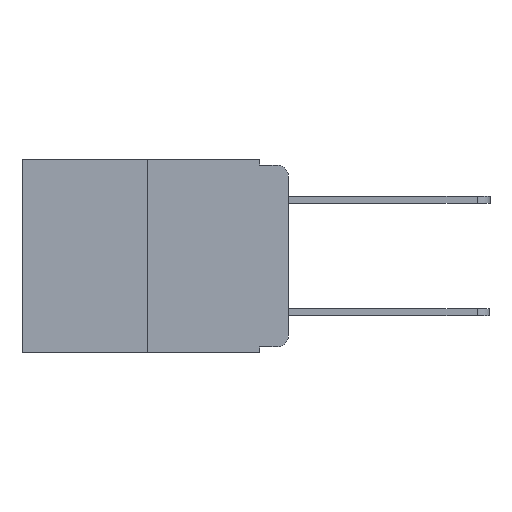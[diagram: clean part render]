
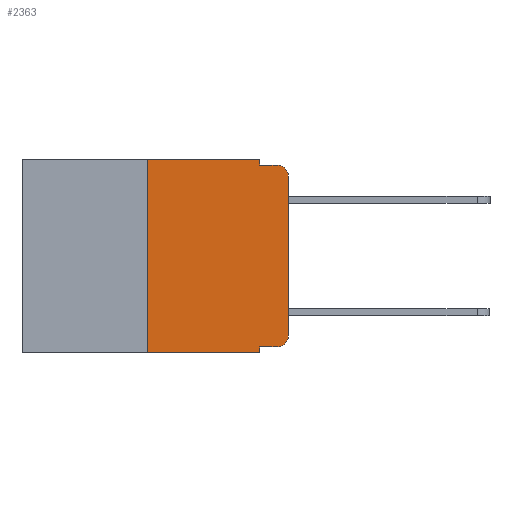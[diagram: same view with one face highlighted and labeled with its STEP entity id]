
A CAD part, left-side view. The second image highlights one B-rep face of the part: STEP entity #2363.
In plain terms, the highlighted planar face has unit normal (-1, 0, 0).
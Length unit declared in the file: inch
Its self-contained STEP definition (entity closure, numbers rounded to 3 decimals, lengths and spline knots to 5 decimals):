
#89 = CARTESIAN_POINT ( 'NONE',  ( 0., 0.051, -0.333 ) ) ;
#152 = ORIENTED_EDGE ( 'NONE', *, *, #4042, .F. ) ;
#178 = DIRECTION ( 'NONE',  ( -1., 0., 0. ) ) ;
#197 = LINE ( 'NONE', #7037, #9937 ) ;
#241 = VECTOR ( 'NONE', #9816, 39.37008 ) ;
#544 = EDGE_CURVE ( 'NONE', #943, #4559, #9463, .T. ) ;
#662 = LINE ( 'NONE', #4929, #1022 ) ;
#840 = CIRCLE ( 'NONE', #10799, 0.02 ) ;
#892 = CARTESIAN_POINT ( 'NONE',  ( 0., 0.473, -0.343 ) ) ;
#908 = CARTESIAN_POINT ( 'NONE',  ( 0., 0.02, -0.333 ) ) ;
#943 = VERTEX_POINT ( 'NONE', #12039 ) ;
#1022 = VECTOR ( 'NONE', #5975, 39.37008 ) ;
#1100 = VERTEX_POINT ( 'NONE', #9265 ) ;
#1186 = VERTEX_POINT ( 'NONE', #7700 ) ;
#1202 = VERTEX_POINT ( 'NONE', #908 ) ;
#1264 = EDGE_CURVE ( 'NONE', #10830, #1186, #840, .T. ) ;
#1956 = DIRECTION ( 'NONE',  ( 0., 0., -1. ) ) ;
#2053 = CARTESIAN_POINT ( 'NONE',  ( 0., 0., -0.313 ) ) ;
#2106 = VECTOR ( 'NONE', #7248, 39.37008 ) ;
#2107 = DIRECTION ( 'NONE',  ( 0., 0., 1. ) ) ;
#2241 = CARTESIAN_POINT ( 'NONE',  ( 0., 0.02, -0.03 ) ) ;
#2311 = VECTOR ( 'NONE', #10447, 39.37008 ) ;
#2363 = ADVANCED_FACE ( 'NONE', ( #5228 ), #12243, .F. ) ;
#2385 = EDGE_CURVE ( 'NONE', #7350, #4559, #12242, .T. ) ;
#2438 = DIRECTION ( 'NONE',  ( 0., 0., 1. ) ) ;
#2677 = ORIENTED_EDGE ( 'NONE', *, *, #10457, .T. ) ;
#2814 = CARTESIAN_POINT ( 'NONE',  ( 0., 0.051, 0. ) ) ;
#2967 = ORIENTED_EDGE ( 'NONE', *, *, #4863, .F. ) ;
#3004 = CARTESIAN_POINT ( 'NONE',  ( 0., 0., -0.03 ) ) ;
#3276 = ORIENTED_EDGE ( 'NONE', *, *, #10829, .T. ) ;
#3390 = DIRECTION ( 'NONE',  ( 0., -1., 0. ) ) ;
#3733 = VERTEX_POINT ( 'NONE', #10480 ) ;
#3808 = VERTEX_POINT ( 'NONE', #2053 ) ;
#3965 = EDGE_CURVE ( 'NONE', #943, #1202, #10266, .T. ) ;
#4001 = ORIENTED_EDGE ( 'NONE', *, *, #544, .F. ) ;
#4042 = EDGE_CURVE ( 'NONE', #3733, #5033, #4704, .T. ) ;
#4559 = VERTEX_POINT ( 'NONE', #4950 ) ;
#4704 = LINE ( 'NONE', #8145, #2106 ) ;
#4743 = DIRECTION ( 'NONE',  ( -1., 0., 0. ) ) ;
#4863 = EDGE_CURVE ( 'NONE', #1100, #3733, #7452, .T. ) ;
#4888 = CARTESIAN_POINT ( 'NONE',  ( 0., 0.473, 0. ) ) ;
#4929 = CARTESIAN_POINT ( 'NONE',  ( 0., 0.051, -0.01 ) ) ;
#4950 = CARTESIAN_POINT ( 'NONE',  ( 0., 0.051, -0.343 ) ) ;
#5033 = VERTEX_POINT ( 'NONE', #5671 ) ;
#5228 = FACE_OUTER_BOUND ( 'NONE', #5438, .T. ) ;
#5269 = ORIENTED_EDGE ( 'NONE', *, *, #12322, .F. ) ;
#5438 = EDGE_LOOP ( 'NONE', ( #2677, #7539, #5269, #152, #2967, #8085, #8780, #4001, #7242, #3276 ) ) ;
#5595 = DIRECTION ( 'NONE',  ( 0., 0., -1. ) ) ;
#5671 = CARTESIAN_POINT ( 'NONE',  ( 0., 0.051, -0.01 ) ) ;
#5767 = LINE ( 'NONE', #8212, #6094 ) ;
#5975 = DIRECTION ( 'NONE',  ( 0., -1., 0. ) ) ;
#6094 = VECTOR ( 'NONE', #2438, 39.37008 ) ;
#6376 = CARTESIAN_POINT ( 'NONE',  ( 0., 0.473, 0. ) ) ;
#6902 = DIRECTION ( 'NONE',  ( 0., 0., -1. ) ) ;
#7037 = CARTESIAN_POINT ( 'NONE',  ( 0., 0., 0. ) ) ;
#7242 = ORIENTED_EDGE ( 'NONE', *, *, #3965, .T. ) ;
#7248 = DIRECTION ( 'NONE',  ( 0., 0., -1. ) ) ;
#7350 = VERTEX_POINT ( 'NONE', #8929 ) ;
#7452 = LINE ( 'NONE', #6376, #11904 ) ;
#7539 = ORIENTED_EDGE ( 'NONE', *, *, #1264, .T. ) ;
#7700 = CARTESIAN_POINT ( 'NONE',  ( 0., 0.02, -0.01 ) ) ;
#7986 = CIRCLE ( 'NONE', #11309, 0.02 ) ;
#8085 = ORIENTED_EDGE ( 'NONE', *, *, #11654, .F. ) ;
#8145 = CARTESIAN_POINT ( 'NONE',  ( 0., 0.051, 0. ) ) ;
#8212 = CARTESIAN_POINT ( 'NONE',  ( 0., 0.25, 0. ) ) ;
#8780 = ORIENTED_EDGE ( 'NONE', *, *, #2385, .T. ) ;
#8929 = CARTESIAN_POINT ( 'NONE',  ( 0., 0.25, -0.343 ) ) ;
#9265 = CARTESIAN_POINT ( 'NONE',  ( 0., 0.25, 0. ) ) ;
#9463 = LINE ( 'NONE', #2814, #11547 ) ;
#9551 = DIRECTION ( 'NONE',  ( 1., 0., 0. ) ) ;
#9816 = DIRECTION ( 'NONE',  ( 0., -1., 0. ) ) ;
#9937 = VECTOR ( 'NONE', #2107, 39.37008 ) ;
#10266 = LINE ( 'NONE', #89, #241 ) ;
#10342 = CARTESIAN_POINT ( 'NONE',  ( 0., 0.02, -0.313 ) ) ;
#10447 = DIRECTION ( 'NONE',  ( 0., -1., 0. ) ) ;
#10457 = EDGE_CURVE ( 'NONE', #3808, #10830, #197, .T. ) ;
#10480 = CARTESIAN_POINT ( 'NONE',  ( 0., 0.051, 0. ) ) ;
#10799 = AXIS2_PLACEMENT_3D ( 'NONE', #2241, #178, #1956 ) ;
#10829 = EDGE_CURVE ( 'NONE', #1202, #3808, #7986, .T. ) ;
#10830 = VERTEX_POINT ( 'NONE', #3004 ) ;
#11205 = DIRECTION ( 'NONE',  ( 0., 0., -1. ) ) ;
#11309 = AXIS2_PLACEMENT_3D ( 'NONE', #10342, #4743, #11205 ) ;
#11325 = AXIS2_PLACEMENT_3D ( 'NONE', #4888, #9551, #6902 ) ;
#11547 = VECTOR ( 'NONE', #5595, 39.37008 ) ;
#11654 = EDGE_CURVE ( 'NONE', #7350, #1100, #5767, .T. ) ;
#11904 = VECTOR ( 'NONE', #3390, 39.37008 ) ;
#12039 = CARTESIAN_POINT ( 'NONE',  ( 0., 0.051, -0.333 ) ) ;
#12242 = LINE ( 'NONE', #892, #2311 ) ;
#12243 = PLANE ( 'NONE',  #11325 ) ;
#12322 = EDGE_CURVE ( 'NONE', #5033, #1186, #662, .T. ) ;
